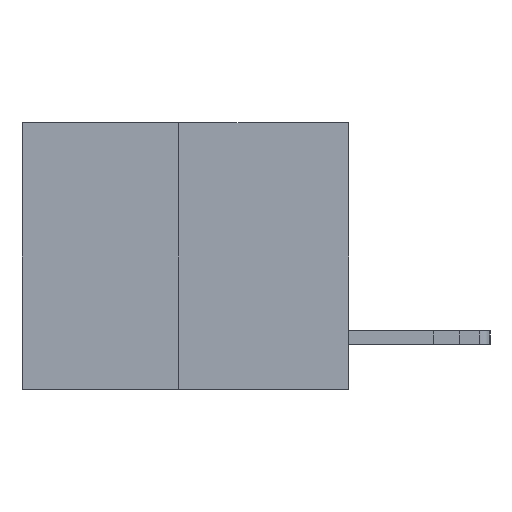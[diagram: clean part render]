
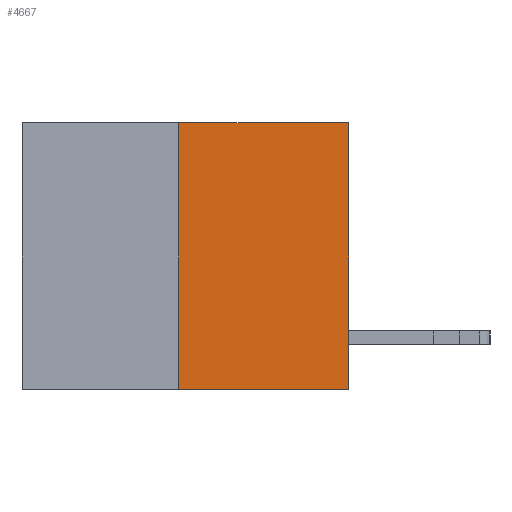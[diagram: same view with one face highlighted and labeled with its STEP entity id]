
A CAD part, left-side view. The second image highlights one B-rep face of the part: STEP entity #4667.
In plain terms, the highlighted planar face has unit normal (-1, 0, 0).
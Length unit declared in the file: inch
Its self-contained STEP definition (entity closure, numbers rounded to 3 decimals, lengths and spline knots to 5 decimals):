
#681 = LINE ( 'NONE', #3625, #2139 ) ;
#836 = CARTESIAN_POINT ( 'NONE',  ( 0., 0., -0.49 ) ) ;
#1533 = DIRECTION ( 'NONE',  ( 0., -1., 0. ) ) ;
#1924 = DIRECTION ( 'NONE',  ( 1., 0., 0. ) ) ;
#2139 = VECTOR ( 'NONE', #1533, 39.37008 ) ;
#2308 = VECTOR ( 'NONE', #14057, 39.37008 ) ;
#2355 = LINE ( 'NONE', #6986, #9337 ) ;
#2913 = AXIS2_PLACEMENT_3D ( 'NONE', #5248, #1924, #14793 ) ;
#3491 = CARTESIAN_POINT ( 'NONE',  ( 0., 0.312, -0.49 ) ) ;
#3625 = CARTESIAN_POINT ( 'NONE',  ( 0., 0.6, 0. ) ) ;
#4131 = LINE ( 'NONE', #6929, #2308 ) ;
#4228 = ORIENTED_EDGE ( 'NONE', *, *, #12042, .F. ) ;
#4667 = ADVANCED_FACE ( 'NONE', ( #4907 ), #12379, .F. ) ;
#4907 = FACE_OUTER_BOUND ( 'NONE', #10863, .T. ) ;
#5248 = CARTESIAN_POINT ( 'NONE',  ( 0., 0.6, 0. ) ) ;
#5513 = DIRECTION ( 'NONE',  ( 0., -1., 0. ) ) ;
#5588 = LINE ( 'NONE', #8916, #6346 ) ;
#5914 = DIRECTION ( 'NONE',  ( 0., 0., 1. ) ) ;
#5924 = EDGE_CURVE ( 'NONE', #6522, #10856, #4131, .T. ) ;
#6124 = VERTEX_POINT ( 'NONE', #3491 ) ;
#6346 = VECTOR ( 'NONE', #5513, 39.37008 ) ;
#6522 = VERTEX_POINT ( 'NONE', #836 ) ;
#6929 = CARTESIAN_POINT ( 'NONE',  ( 0., 0., 0. ) ) ;
#6956 = ORIENTED_EDGE ( 'NONE', *, *, #7042, .F. ) ;
#6986 = CARTESIAN_POINT ( 'NONE',  ( 0., 0.312, -0.49 ) ) ;
#7042 = EDGE_CURVE ( 'NONE', #8730, #10856, #681, .T. ) ;
#8443 = CARTESIAN_POINT ( 'NONE',  ( 0., 0., 0. ) ) ;
#8631 = CARTESIAN_POINT ( 'NONE',  ( 0., 0.312, 0. ) ) ;
#8730 = VERTEX_POINT ( 'NONE', #8631 ) ;
#8916 = CARTESIAN_POINT ( 'NONE',  ( 0., 0.6, -0.49 ) ) ;
#9337 = VECTOR ( 'NONE', #5914, 39.37008 ) ;
#10480 = ORIENTED_EDGE ( 'NONE', *, *, #14123, .T. ) ;
#10856 = VERTEX_POINT ( 'NONE', #8443 ) ;
#10863 = EDGE_LOOP ( 'NONE', ( #4228, #10480, #12485, #6956 ) ) ;
#12042 = EDGE_CURVE ( 'NONE', #6124, #8730, #2355, .T. ) ;
#12379 = PLANE ( 'NONE',  #2913 ) ;
#12485 = ORIENTED_EDGE ( 'NONE', *, *, #5924, .T. ) ;
#14057 = DIRECTION ( 'NONE',  ( 0., 0., 1. ) ) ;
#14123 = EDGE_CURVE ( 'NONE', #6124, #6522, #5588, .T. ) ;
#14793 = DIRECTION ( 'NONE',  ( 0., 0., -1. ) ) ;
